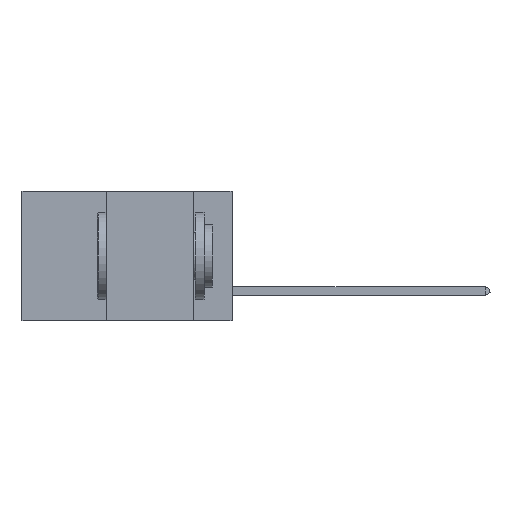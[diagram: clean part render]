
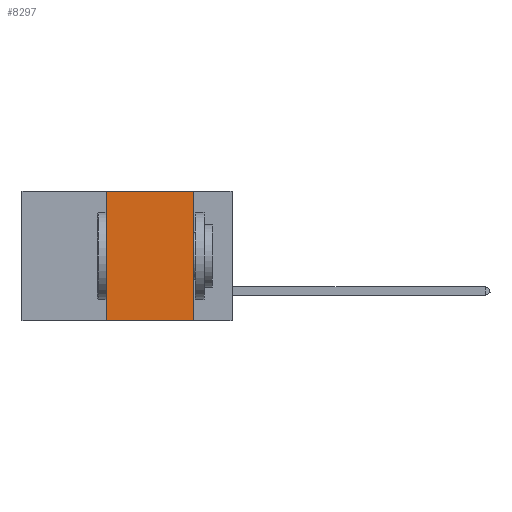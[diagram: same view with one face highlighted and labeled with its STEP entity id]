
A CAD part, left-side view. The second image highlights one B-rep face of the part: STEP entity #8297.
In plain terms, the highlighted planar face has unit normal (-1, 0, 0).
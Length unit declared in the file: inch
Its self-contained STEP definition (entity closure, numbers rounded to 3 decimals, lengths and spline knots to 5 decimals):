
#33 = ORIENTED_EDGE ( 'NONE', *, *, #22937, .F. ) ;
#193 = CARTESIAN_POINT ( 'NONE',  ( 0., 0.6, 0. ) ) ;
#443 = VECTOR ( 'NONE', #19768, 39.37008 ) ;
#453 = VERTEX_POINT ( 'NONE', #14226 ) ;
#501 = VERTEX_POINT ( 'NONE', #11929 ) ;
#864 = DIRECTION ( 'NONE',  ( 0., 0., -1. ) ) ;
#1843 = CARTESIAN_POINT ( 'NONE',  ( 0., 0.6, 0. ) ) ;
#2988 = LINE ( 'NONE', #13537, #10540 ) ;
#4083 = VERTEX_POINT ( 'NONE', #6406 ) ;
#5545 = LINE ( 'NONE', #9434, #23393 ) ;
#5584 = DIRECTION ( 'NONE',  ( 0., 0., 1. ) ) ;
#6406 = CARTESIAN_POINT ( 'NONE',  ( 0., 0.11, -0.37 ) ) ;
#8297 = ADVANCED_FACE ( 'NONE', ( #14929 ), #12263, .F. ) ;
#8904 = LINE ( 'NONE', #14765, #12988 ) ;
#8923 = EDGE_CURVE ( 'NONE', #501, #22735, #21160, .T. ) ;
#8964 = EDGE_CURVE ( 'NONE', #453, #501, #2988, .T. ) ;
#9223 = ORIENTED_EDGE ( 'NONE', *, *, #8964, .F. ) ;
#9434 = CARTESIAN_POINT ( 'NONE',  ( 0., 0.6, -0.37 ) ) ;
#10540 = VECTOR ( 'NONE', #5584, 39.37008 ) ;
#11929 = CARTESIAN_POINT ( 'NONE',  ( 0., 0.36, 0. ) ) ;
#12263 = PLANE ( 'NONE',  #22090 ) ;
#12988 = VECTOR ( 'NONE', #25138, 39.37008 ) ;
#13537 = CARTESIAN_POINT ( 'NONE',  ( 0., 0.36, 0. ) ) ;
#14226 = CARTESIAN_POINT ( 'NONE',  ( 0., 0.36, -0.37 ) ) ;
#14739 = ORIENTED_EDGE ( 'NONE', *, *, #8923, .F. ) ;
#14765 = CARTESIAN_POINT ( 'NONE',  ( 0., 0.11, 0. ) ) ;
#14929 = FACE_OUTER_BOUND ( 'NONE', #19103, .T. ) ;
#16447 = CARTESIAN_POINT ( 'NONE',  ( 0., 0.11, 0. ) ) ;
#16815 = ORIENTED_EDGE ( 'NONE', *, *, #22103, .T. ) ;
#18386 = DIRECTION ( 'NONE',  ( 1., 0., 0. ) ) ;
#19103 = EDGE_LOOP ( 'NONE', ( #33, #14739, #9223, #16815 ) ) ;
#19768 = DIRECTION ( 'NONE',  ( 0., -1., 0. ) ) ;
#21160 = LINE ( 'NONE', #1843, #443 ) ;
#22090 = AXIS2_PLACEMENT_3D ( 'NONE', #193, #18386, #864 ) ;
#22103 = EDGE_CURVE ( 'NONE', #453, #4083, #5545, .T. ) ;
#22735 = VERTEX_POINT ( 'NONE', #16447 ) ;
#22937 = EDGE_CURVE ( 'NONE', #22735, #4083, #8904, .T. ) ;
#23393 = VECTOR ( 'NONE', #25229, 39.37008 ) ;
#25138 = DIRECTION ( 'NONE',  ( 0., 0., -1. ) ) ;
#25229 = DIRECTION ( 'NONE',  ( 0., -1., 0. ) ) ;
